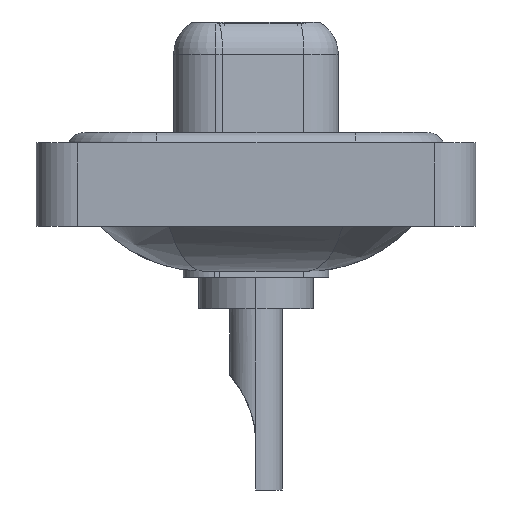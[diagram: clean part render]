
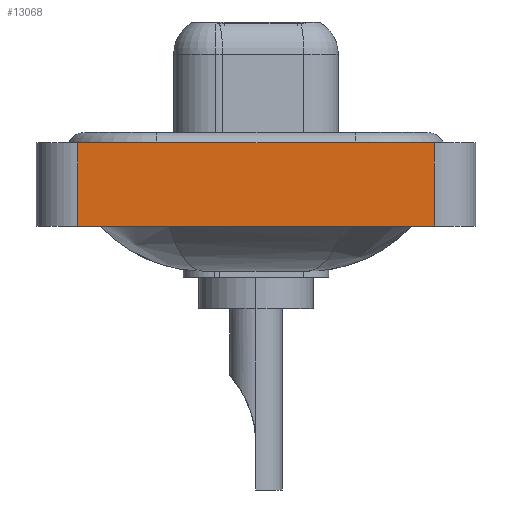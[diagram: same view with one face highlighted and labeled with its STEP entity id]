
A CAD part, left-side view. The second image highlights one B-rep face of the part: STEP entity #13068.
In plain terms, the highlighted planar face has unit normal (-1, 0, 0).
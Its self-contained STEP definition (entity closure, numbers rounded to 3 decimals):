
#37 = DIRECTION ( 'NONE',  ( 0., 0., 1. ) ) ;
#154 = VERTEX_POINT ( 'NONE', #1731 ) ;
#245 = DIRECTION ( 'NONE',  ( 0., -1., 0. ) ) ;
#1115 = ORIENTED_EDGE ( 'NONE', *, *, #9657, .T. ) ;
#1252 = CARTESIAN_POINT ( 'NONE',  ( -7.3, 8.55, -3.6 ) ) ;
#1731 = CARTESIAN_POINT ( 'NONE',  ( -7.3, -8.55, -3.6 ) ) ;
#1780 = DIRECTION ( 'NONE',  ( -1., 0., 0. ) ) ;
#2219 = LINE ( 'NONE', #13427, #7256 ) ;
#2479 = LINE ( 'NONE', #1252, #12219 ) ;
#2601 = CARTESIAN_POINT ( 'NONE',  ( -7.3, -8.55, -3.6 ) ) ;
#3315 = ORIENTED_EDGE ( 'NONE', *, *, #8516, .T. ) ;
#3619 = EDGE_CURVE ( 'NONE', #7422, #7055, #7727, .T. ) ;
#4125 = EDGE_LOOP ( 'NONE', ( #1115, #12130, #8669, #3315 ) ) ;
#5953 = VECTOR ( 'NONE', #6411, 1000. ) ;
#6236 = EDGE_CURVE ( 'NONE', #7592, #7422, #2479, .T. ) ;
#6411 = DIRECTION ( 'NONE',  ( 0., -1., 0. ) ) ;
#6751 = DIRECTION ( 'NONE',  ( 0., 0., 1. ) ) ;
#7055 = VERTEX_POINT ( 'NONE', #12368 ) ;
#7256 = VECTOR ( 'NONE', #14591, 1000. ) ;
#7422 = VERTEX_POINT ( 'NONE', #13077 ) ;
#7585 = CARTESIAN_POINT ( 'NONE',  ( -7.3, -8.55, 0.4 ) ) ;
#7592 = VERTEX_POINT ( 'NONE', #10062 ) ;
#7727 = LINE ( 'NONE', #7585, #12411 ) ;
#8516 = EDGE_CURVE ( 'NONE', #7592, #154, #8860, .T. ) ;
#8669 = ORIENTED_EDGE ( 'NONE', *, *, #6236, .F. ) ;
#8860 = LINE ( 'NONE', #2601, #5953 ) ;
#9657 = EDGE_CURVE ( 'NONE', #154, #7055, #2219, .T. ) ;
#9908 = AXIS2_PLACEMENT_3D ( 'NONE', #15298, #1780, #6751 ) ;
#10062 = CARTESIAN_POINT ( 'NONE',  ( -7.3, 8.55, -3.6 ) ) ;
#10329 = FACE_OUTER_BOUND ( 'NONE', #4125, .T. ) ;
#12130 = ORIENTED_EDGE ( 'NONE', *, *, #3619, .F. ) ;
#12219 = VECTOR ( 'NONE', #37, 1000. ) ;
#12368 = CARTESIAN_POINT ( 'NONE',  ( -7.3, -8.55, 0.4 ) ) ;
#12411 = VECTOR ( 'NONE', #245, 1000. ) ;
#12923 = PLANE ( 'NONE',  #9908 ) ;
#13068 = ADVANCED_FACE ( 'NONE', ( #10329 ), #12923, .T. ) ;
#13077 = CARTESIAN_POINT ( 'NONE',  ( -7.3, 8.55, 0.4 ) ) ;
#13427 = CARTESIAN_POINT ( 'NONE',  ( -7.3, -8.55, -3.6 ) ) ;
#14591 = DIRECTION ( 'NONE',  ( 0., 0., 1. ) ) ;
#15298 = CARTESIAN_POINT ( 'NONE',  ( -7.3, -8.55, -3.6 ) ) ;
